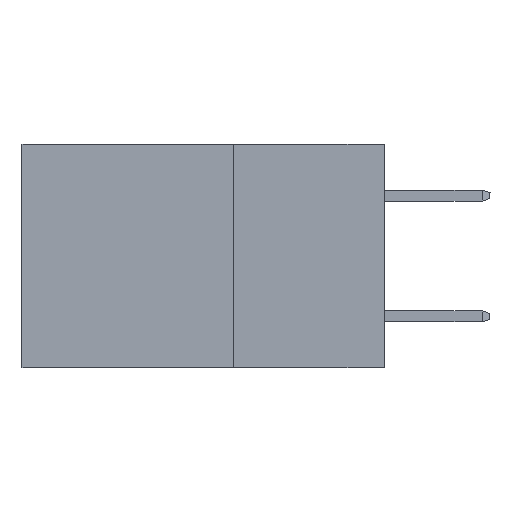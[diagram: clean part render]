
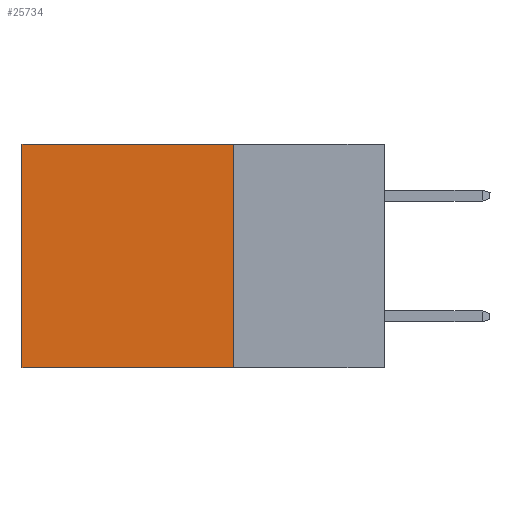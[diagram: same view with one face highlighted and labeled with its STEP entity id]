
A CAD part, left-side view. The second image highlights one B-rep face of the part: STEP entity #25734.
In plain terms, the highlighted planar face has unit normal (-1, 0, 0).
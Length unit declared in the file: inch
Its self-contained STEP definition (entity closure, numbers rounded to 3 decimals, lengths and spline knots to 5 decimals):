
#134 = DIRECTION ( 'NONE',  ( 0., 0., -1. ) ) ;
#671 = VECTOR ( 'NONE', #16852, 39.37008 ) ;
#901 = VECTOR ( 'NONE', #20243, 39.37008 ) ;
#1394 = CARTESIAN_POINT ( 'NONE',  ( 0.298, 0.25, 0. ) ) ;
#3161 = VERTEX_POINT ( 'NONE', #11412 ) ;
#3182 = EDGE_CURVE ( 'NONE', #3161, #21148, #23329, .T. ) ;
#3540 = EDGE_CURVE ( 'NONE', #4803, #10531, #25424, .T. ) ;
#4803 = VERTEX_POINT ( 'NONE', #1394 ) ;
#6847 = CARTESIAN_POINT ( 'NONE',  ( 0.298, 0.25, 0. ) ) ;
#7668 = ORIENTED_EDGE ( 'NONE', *, *, #3182, .T. ) ;
#9696 = FACE_OUTER_BOUND ( 'NONE', #16022, .T. ) ;
#10531 = VERTEX_POINT ( 'NONE', #26404 ) ;
#11412 = CARTESIAN_POINT ( 'NONE',  ( 0.298, 0.6, 0. ) ) ;
#11579 = DIRECTION ( 'NONE',  ( 1., 0., 0. ) ) ;
#12849 = VECTOR ( 'NONE', #30010, 39.37008 ) ;
#15694 = AXIS2_PLACEMENT_3D ( 'NONE', #25471, #11579, #27774 ) ;
#16022 = EDGE_LOOP ( 'NONE', ( #7668, #19782, #27204, #27109 ) ) ;
#16058 = CARTESIAN_POINT ( 'NONE',  ( 0.298, 0.6, -0.37 ) ) ;
#16130 = PLANE ( 'NONE',  #15694 ) ;
#16852 = DIRECTION ( 'NONE',  ( 0., 0., -1. ) ) ;
#17901 = CARTESIAN_POINT ( 'NONE',  ( 0.298, 0.25, -0.37 ) ) ;
#19088 = LINE ( 'NONE', #29918, #12849 ) ;
#19531 = LINE ( 'NONE', #17901, #901 ) ;
#19633 = CARTESIAN_POINT ( 'NONE',  ( 0.298, 0.6, 0. ) ) ;
#19782 = ORIENTED_EDGE ( 'NONE', *, *, #28290, .F. ) ;
#20243 = DIRECTION ( 'NONE',  ( 0., 1., 0. ) ) ;
#21148 = VERTEX_POINT ( 'NONE', #16058 ) ;
#22613 = VECTOR ( 'NONE', #134, 39.37008 ) ;
#23329 = LINE ( 'NONE', #19633, #22613 ) ;
#25424 = LINE ( 'NONE', #6847, #671 ) ;
#25471 = CARTESIAN_POINT ( 'NONE',  ( 0.298, 0.25, 0. ) ) ;
#25734 = ADVANCED_FACE ( 'NONE', ( #9696 ), #16130, .F. ) ;
#26404 = CARTESIAN_POINT ( 'NONE',  ( 0.298, 0.25, -0.37 ) ) ;
#26935 = EDGE_CURVE ( 'NONE', #4803, #3161, #19088, .T. ) ;
#27109 = ORIENTED_EDGE ( 'NONE', *, *, #26935, .T. ) ;
#27204 = ORIENTED_EDGE ( 'NONE', *, *, #3540, .F. ) ;
#27774 = DIRECTION ( 'NONE',  ( 0., 0., -1. ) ) ;
#28290 = EDGE_CURVE ( 'NONE', #10531, #21148, #19531, .T. ) ;
#29918 = CARTESIAN_POINT ( 'NONE',  ( 0.298, 0.25, 0. ) ) ;
#30010 = DIRECTION ( 'NONE',  ( 0., 1., 0. ) ) ;
